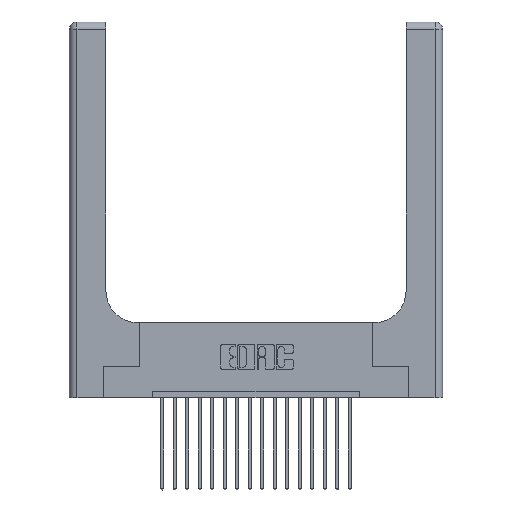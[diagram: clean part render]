
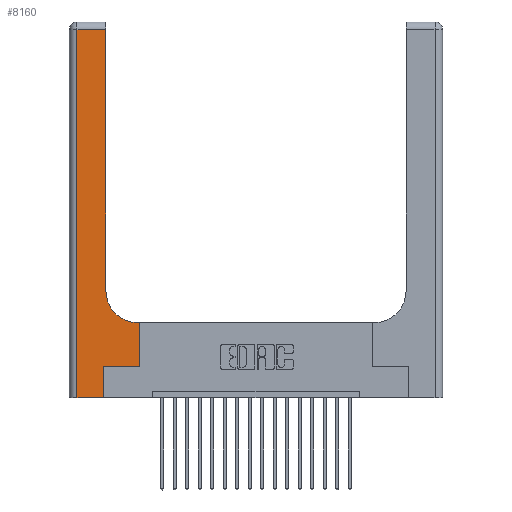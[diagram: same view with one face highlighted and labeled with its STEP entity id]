
A CAD part, top view. The second image highlights one B-rep face of the part: STEP entity #8160.
In plain terms, the highlighted planar face has unit normal (0, 0, 1).
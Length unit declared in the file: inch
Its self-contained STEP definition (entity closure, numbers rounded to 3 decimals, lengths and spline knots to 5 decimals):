
#84 = DIRECTION ( 'NONE',  ( -1., 0., 0. ) ) ;
#282 = DIRECTION ( 'NONE',  ( -1., 0., 0. ) ) ;
#790 = DIRECTION ( 'NONE',  ( 0., 1., 0. ) ) ;
#840 = CARTESIAN_POINT ( 'NONE',  ( 0.5585, 0.6, 0.37 ) ) ;
#893 = CARTESIAN_POINT ( 'NONE',  ( 0.269, 0.25, 0.37 ) ) ;
#956 = CARTESIAN_POINT ( 'NONE',  ( 0.06, 0., 0.37 ) ) ;
#1034 = CARTESIAN_POINT ( 'NONE',  ( 0.5585, 0.25, 0.37 ) ) ;
#1212 = ORIENTED_EDGE ( 'NONE', *, *, #16757, .T. ) ;
#1383 = EDGE_CURVE ( 'NONE', #7340, #8150, #10739, .T. ) ;
#1443 = AXIS2_PLACEMENT_3D ( 'NONE', #15238, #2253, #13454 ) ;
#1604 = VECTOR ( 'NONE', #7558, 39.37008 ) ;
#1625 = CARTESIAN_POINT ( 'NONE',  ( 0., 0., 0.37 ) ) ;
#1757 = VERTEX_POINT ( 'NONE', #893 ) ;
#2253 = DIRECTION ( 'NONE',  ( 0., 0., -1. ) ) ;
#2896 = VERTEX_POINT ( 'NONE', #956 ) ;
#3251 = VECTOR ( 'NONE', #84, 39.37008 ) ;
#3329 = CARTESIAN_POINT ( 'NONE',  ( 0.2915, 2.94, 0.37 ) ) ;
#3634 = VECTOR ( 'NONE', #17267, 39.37008 ) ;
#3867 = EDGE_CURVE ( 'NONE', #8150, #16201, #19244, .T. ) ;
#4406 = LINE ( 'NONE', #5813, #14975 ) ;
#4741 = CARTESIAN_POINT ( 'NONE',  ( 0.5415, 0.85, 0.37 ) ) ;
#4950 = ORIENTED_EDGE ( 'NONE', *, *, #16086, .T. ) ;
#5239 = ORIENTED_EDGE ( 'NONE', *, *, #3867, .T. ) ;
#5790 = LINE ( 'NONE', #6505, #9316 ) ;
#5813 = CARTESIAN_POINT ( 'NONE',  ( 0.269, 0., 0.37 ) ) ;
#6043 = CARTESIAN_POINT ( 'NONE',  ( 0.269, 0.25, 0.37 ) ) ;
#6068 = ORIENTED_EDGE ( 'NONE', *, *, #15945, .T. ) ;
#6400 = CARTESIAN_POINT ( 'NONE',  ( 0.5585, 0.25, 0.37 ) ) ;
#6471 = VECTOR ( 'NONE', #13943, 39.37008 ) ;
#6505 = CARTESIAN_POINT ( 'NONE',  ( 0.06, 3., 0.37 ) ) ;
#7154 = PLANE ( 'NONE',  #1443 ) ;
#7340 = VERTEX_POINT ( 'NONE', #6400 ) ;
#7558 = DIRECTION ( 'NONE',  ( 0., 1., 0. ) ) ;
#7631 = VECTOR ( 'NONE', #12653, 39.37008 ) ;
#8150 = VERTEX_POINT ( 'NONE', #840 ) ;
#8160 = ADVANCED_FACE ( 'NONE', ( #10773 ), #7154, .F. ) ;
#8430 = CARTESIAN_POINT ( 'NONE',  ( 0.06, 2.94, 0.37 ) ) ;
#8515 = VERTEX_POINT ( 'NONE', #8430 ) ;
#9282 = CIRCLE ( 'NONE', #19103, 0.25 ) ;
#9316 = VECTOR ( 'NONE', #17719, 39.37008 ) ;
#9885 = LINE ( 'NONE', #1625, #7631 ) ;
#10118 = VERTEX_POINT ( 'NONE', #11643 ) ;
#10344 = ORIENTED_EDGE ( 'NONE', *, *, #1383, .T. ) ;
#10739 = LINE ( 'NONE', #1034, #6471 ) ;
#10773 = FACE_OUTER_BOUND ( 'NONE', #12200, .T. ) ;
#11406 = DIRECTION ( 'NONE',  ( 0., 0., -1. ) ) ;
#11643 = CARTESIAN_POINT ( 'NONE',  ( 0.2915, 0.85, 0.37 ) ) ;
#11897 = EDGE_CURVE ( 'NONE', #8515, #2896, #5790, .T. ) ;
#12200 = EDGE_LOOP ( 'NONE', ( #12839, #6068, #13098, #1212, #4950, #19279, #10344, #5239, #13117 ) ) ;
#12653 = DIRECTION ( 'NONE',  ( 1., 0., 0. ) ) ;
#12697 = CARTESIAN_POINT ( 'NONE',  ( 0., 2.94, 0.37 ) ) ;
#12839 = ORIENTED_EDGE ( 'NONE', *, *, #17297, .T. ) ;
#13098 = ORIENTED_EDGE ( 'NONE', *, *, #11897, .T. ) ;
#13117 = ORIENTED_EDGE ( 'NONE', *, *, #13250, .T. ) ;
#13250 = EDGE_CURVE ( 'NONE', #16201, #10118, #9282, .T. ) ;
#13454 = DIRECTION ( 'NONE',  ( -1., 0., 0. ) ) ;
#13815 = LINE ( 'NONE', #12697, #3251 ) ;
#13943 = DIRECTION ( 'NONE',  ( 0., 1., 0. ) ) ;
#14076 = CARTESIAN_POINT ( 'NONE',  ( 0.269, 0., 0.37 ) ) ;
#14816 = VERTEX_POINT ( 'NONE', #3329 ) ;
#14975 = VECTOR ( 'NONE', #790, 39.37008 ) ;
#15010 = VECTOR ( 'NONE', #282, 39.37008 ) ;
#15058 = VERTEX_POINT ( 'NONE', #14076 ) ;
#15238 = CARTESIAN_POINT ( 'NONE',  ( 0., 3., 0.37 ) ) ;
#15652 = LINE ( 'NONE', #17317, #1604 ) ;
#15945 = EDGE_CURVE ( 'NONE', #14816, #8515, #13815, .T. ) ;
#16086 = EDGE_CURVE ( 'NONE', #15058, #1757, #4406, .T. ) ;
#16201 = VERTEX_POINT ( 'NONE', #20200 ) ;
#16595 = EDGE_CURVE ( 'NONE', #1757, #7340, #17931, .T. ) ;
#16757 = EDGE_CURVE ( 'NONE', #2896, #15058, #9885, .T. ) ;
#17267 = DIRECTION ( 'NONE',  ( 1., 0., 0. ) ) ;
#17297 = EDGE_CURVE ( 'NONE', #10118, #14816, #15652, .T. ) ;
#17317 = CARTESIAN_POINT ( 'NONE',  ( 0.2915, 3., 0.37 ) ) ;
#17719 = DIRECTION ( 'NONE',  ( 0., -1., 0. ) ) ;
#17931 = LINE ( 'NONE', #6043, #3634 ) ;
#19103 = AXIS2_PLACEMENT_3D ( 'NONE', #4741, #11406, #19329 ) ;
#19244 = LINE ( 'NONE', #20615, #15010 ) ;
#19279 = ORIENTED_EDGE ( 'NONE', *, *, #16595, .T. ) ;
#19329 = DIRECTION ( 'NONE',  ( 1., 0., 0. ) ) ;
#20200 = CARTESIAN_POINT ( 'NONE',  ( 0.5415, 0.6, 0.37 ) ) ;
#20615 = CARTESIAN_POINT ( 'NONE',  ( 0.2915, 0.6, 0.37 ) ) ;
